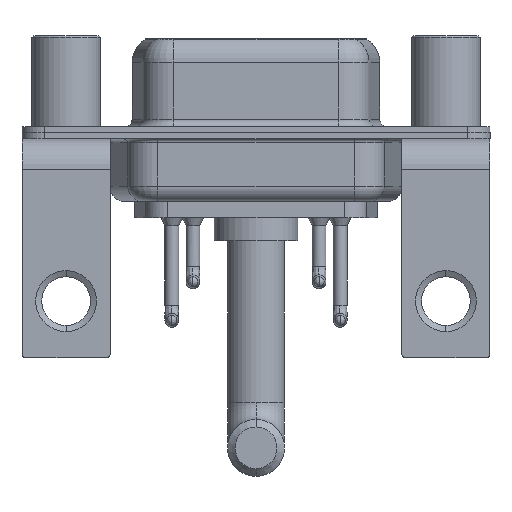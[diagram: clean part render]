
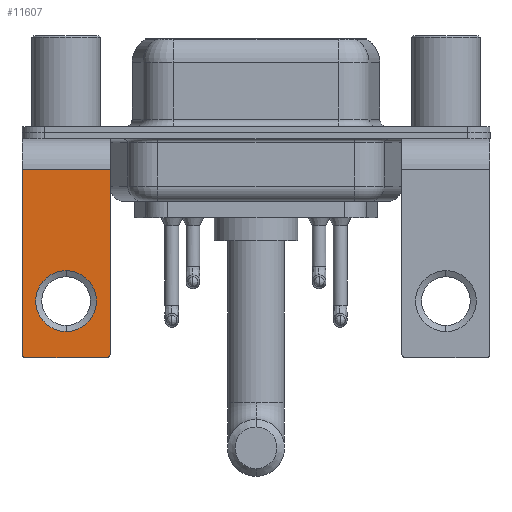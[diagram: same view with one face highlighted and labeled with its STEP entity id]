
A CAD part, front view. The second image highlights one B-rep face of the part: STEP entity #11607.
In plain terms, the highlighted planar face has unit normal (0, -1, 0).
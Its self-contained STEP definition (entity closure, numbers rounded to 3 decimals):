
#82 = CARTESIAN_POINT ( 'NONE',  ( 0., -6.25, -11.07 ) ) ;
#242 = EDGE_CURVE ( 'NONE', #14216, #2020, #14621, .T. ) ;
#244 = DIRECTION ( 'NONE',  ( 0., -1., 0. ) ) ;
#631 = CIRCLE ( 'NONE', #3062, 2. ) ;
#700 = DIRECTION ( 'NONE',  ( -1., 0., 0. ) ) ;
#935 = AXIS2_PLACEMENT_3D ( 'NONE', #11903, #244, #4734 ) ;
#1454 = EDGE_CURVE ( 'NONE', #14296, #3171, #4290, .T. ) ;
#1587 = CARTESIAN_POINT ( 'NONE',  ( 0., -6.25, -13.07 ) ) ;
#1809 = FACE_BOUND ( 'NONE', #7784, .T. ) ;
#2020 = VERTEX_POINT ( 'NONE', #16874 ) ;
#2546 = EDGE_CURVE ( 'NONE', #14216, #8005, #12792, .T. ) ;
#3062 = AXIS2_PLACEMENT_3D ( 'NONE', #82, #6023, #3325 ) ;
#3097 = DIRECTION ( 'NONE',  ( -1., 0., 0. ) ) ;
#3171 = VERTEX_POINT ( 'NONE', #9934 ) ;
#3281 = CARTESIAN_POINT ( 'NONE',  ( 0., -6.25, -9.07 ) ) ;
#3325 = DIRECTION ( 'NONE',  ( 0., 0., 1. ) ) ;
#4238 = DIRECTION ( 'NONE',  ( 0., 1., 0. ) ) ;
#4290 = CIRCLE ( 'NONE', #935, 0.25 ) ;
#4538 = DIRECTION ( 'NONE',  ( 0., -1., 0. ) ) ;
#4658 = VECTOR ( 'NONE', #700, 1000. ) ;
#4734 = DIRECTION ( 'NONE',  ( 0., 0., 1. ) ) ;
#5003 = LINE ( 'NONE', #13767, #4658 ) ;
#5367 = ORIENTED_EDGE ( 'NONE', *, *, #8979, .T. ) ;
#6023 = DIRECTION ( 'NONE',  ( 0., 1., 0. ) ) ;
#6232 = CARTESIAN_POINT ( 'NONE',  ( -2.9, -6.25, -2.4 ) ) ;
#6331 = LINE ( 'NONE', #6232, #17972 ) ;
#6342 = CARTESIAN_POINT ( 'NONE',  ( -2.9, -6.25, -14.55 ) ) ;
#6592 = DIRECTION ( 'NONE',  ( 0., 0., 1. ) ) ;
#6997 = ORIENTED_EDGE ( 'NONE', *, *, #14499, .F. ) ;
#7784 = EDGE_LOOP ( 'NONE', ( #16847, #5367 ) ) ;
#8005 = VERTEX_POINT ( 'NONE', #16770 ) ;
#8006 = ORIENTED_EDGE ( 'NONE', *, *, #2546, .F. ) ;
#8641 = CARTESIAN_POINT ( 'NONE',  ( 2.9, -6.25, -2.4 ) ) ;
#8724 = CARTESIAN_POINT ( 'NONE',  ( 0., -6.25, -11.07 ) ) ;
#8779 = EDGE_LOOP ( 'NONE', ( #13098, #8851, #6997, #12572, #8006, #15802 ) ) ;
#8799 = VERTEX_POINT ( 'NONE', #3281 ) ;
#8851 = ORIENTED_EDGE ( 'NONE', *, *, #1454, .T. ) ;
#8979 = EDGE_CURVE ( 'NONE', #8799, #12448, #631, .T. ) ;
#9313 = CIRCLE ( 'NONE', #12968, 2. ) ;
#9477 = AXIS2_PLACEMENT_3D ( 'NONE', #11801, #4538, #10364 ) ;
#9548 = PLANE ( 'NONE',  #12537 ) ;
#9758 = CARTESIAN_POINT ( 'NONE',  ( 2.9, -6.25, -2.4 ) ) ;
#9838 = VECTOR ( 'NONE', #12702, 1000. ) ;
#9934 = CARTESIAN_POINT ( 'NONE',  ( -2.65, -6.25, -14.8 ) ) ;
#10174 = CARTESIAN_POINT ( 'NONE',  ( 2.65, -6.25, -14.8 ) ) ;
#10364 = DIRECTION ( 'NONE',  ( 0., 0., 1. ) ) ;
#10537 = CARTESIAN_POINT ( 'NONE',  ( 2.9, -6.25, -2.4 ) ) ;
#11355 = DIRECTION ( 'NONE',  ( 0., 1., 0. ) ) ;
#11607 = ADVANCED_FACE ( 'NONE', ( #1809, #12028 ), #9548, .F. ) ;
#11801 = CARTESIAN_POINT ( 'NONE',  ( 2.65, -6.25, -14.55 ) ) ;
#11903 = CARTESIAN_POINT ( 'NONE',  ( -2.65, -6.25, -14.55 ) ) ;
#12028 = FACE_OUTER_BOUND ( 'NONE', #8779, .T. ) ;
#12448 = VERTEX_POINT ( 'NONE', #1587 ) ;
#12525 = CIRCLE ( 'NONE', #9477, 0.25 ) ;
#12537 = AXIS2_PLACEMENT_3D ( 'NONE', #16738, #11355, #6592 ) ;
#12572 = ORIENTED_EDGE ( 'NONE', *, *, #12676, .T. ) ;
#12676 = EDGE_CURVE ( 'NONE', #14125, #8005, #12525, .T. ) ;
#12702 = DIRECTION ( 'NONE',  ( 0., 0., -1. ) ) ;
#12792 = LINE ( 'NONE', #9758, #9838 ) ;
#12968 = AXIS2_PLACEMENT_3D ( 'NONE', #8724, #4238, #13091 ) ;
#13091 = DIRECTION ( 'NONE',  ( 0., 0., 1. ) ) ;
#13098 = ORIENTED_EDGE ( 'NONE', *, *, #13102, .T. ) ;
#13102 = EDGE_CURVE ( 'NONE', #2020, #14296, #6331, .T. ) ;
#13767 = CARTESIAN_POINT ( 'NONE',  ( 2.9, -6.25, -14.8 ) ) ;
#14125 = VERTEX_POINT ( 'NONE', #10174 ) ;
#14216 = VERTEX_POINT ( 'NONE', #10537 ) ;
#14296 = VERTEX_POINT ( 'NONE', #6342 ) ;
#14499 = EDGE_CURVE ( 'NONE', #14125, #3171, #5003, .T. ) ;
#14621 = LINE ( 'NONE', #8641, #17599 ) ;
#14801 = DIRECTION ( 'NONE',  ( 0., 0., -1. ) ) ;
#15802 = ORIENTED_EDGE ( 'NONE', *, *, #242, .T. ) ;
#16738 = CARTESIAN_POINT ( 'NONE',  ( 2.9, -6.25, -2.4 ) ) ;
#16770 = CARTESIAN_POINT ( 'NONE',  ( 2.9, -6.25, -14.55 ) ) ;
#16847 = ORIENTED_EDGE ( 'NONE', *, *, #17491, .T. ) ;
#16874 = CARTESIAN_POINT ( 'NONE',  ( -2.9, -6.25, -2.4 ) ) ;
#17491 = EDGE_CURVE ( 'NONE', #12448, #8799, #9313, .T. ) ;
#17599 = VECTOR ( 'NONE', #3097, 1000. ) ;
#17972 = VECTOR ( 'NONE', #14801, 1000. ) ;
